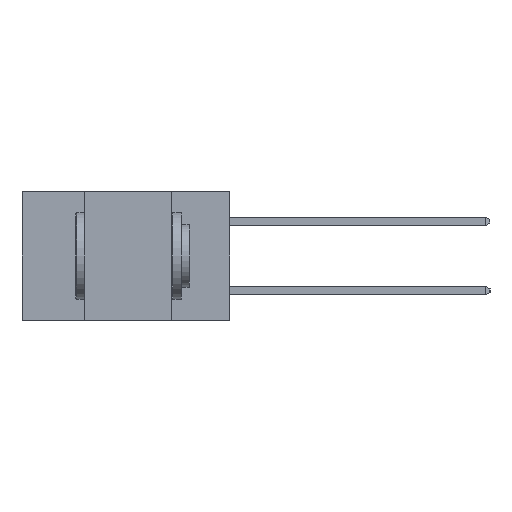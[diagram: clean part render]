
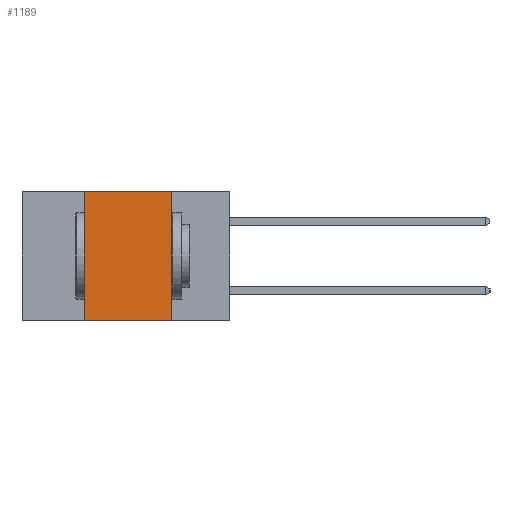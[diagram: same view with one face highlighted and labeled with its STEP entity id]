
A CAD part, left-side view. The second image highlights one B-rep face of the part: STEP entity #1189.
In plain terms, the highlighted planar face has unit normal (-1, 0, 0).
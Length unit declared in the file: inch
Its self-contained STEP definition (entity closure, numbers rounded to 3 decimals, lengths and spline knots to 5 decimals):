
#81 = PLANE ( 'NONE',  #7124 ) ;
#119 = VECTOR ( 'NONE', #3051, 39.37008 ) ;
#1189 = ADVANCED_FACE ( 'NONE', ( #8420 ), #81, .F. ) ;
#1396 = CARTESIAN_POINT ( 'NONE',  ( 0., 0.42, 0. ) ) ;
#1532 = CARTESIAN_POINT ( 'NONE',  ( 0., 0.42, -0.37 ) ) ;
#1767 = CARTESIAN_POINT ( 'NONE',  ( 0., 0.42, -0.37 ) ) ;
#2162 = LINE ( 'NONE', #2356, #16603 ) ;
#2356 = CARTESIAN_POINT ( 'NONE',  ( 0., 0.6, -0.37 ) ) ;
#3051 = DIRECTION ( 'NONE',  ( 0., 0., 1. ) ) ;
#4381 = CARTESIAN_POINT ( 'NONE',  ( 0., 0.17, -0.37 ) ) ;
#4747 = CARTESIAN_POINT ( 'NONE',  ( 0., 0.17, -0.37 ) ) ;
#5087 = LINE ( 'NONE', #9373, #15148 ) ;
#5851 = DIRECTION ( 'NONE',  ( 0., 0., -1. ) ) ;
#5996 = VERTEX_POINT ( 'NONE', #1767 ) ;
#7124 = AXIS2_PLACEMENT_3D ( 'NONE', #9971, #8505, #9987 ) ;
#7237 = VERTEX_POINT ( 'NONE', #1396 ) ;
#8259 = LINE ( 'NONE', #4381, #15367 ) ;
#8420 = FACE_OUTER_BOUND ( 'NONE', #13849, .T. ) ;
#8505 = DIRECTION ( 'NONE',  ( 1., 0., 0. ) ) ;
#8555 = EDGE_CURVE ( 'NONE', #5996, #16968, #2162, .T. ) ;
#8582 = ORIENTED_EDGE ( 'NONE', *, *, #8555, .T. ) ;
#8781 = ORIENTED_EDGE ( 'NONE', *, *, #18236, .F. ) ;
#8839 = ORIENTED_EDGE ( 'NONE', *, *, #16520, .F. ) ;
#8929 = ORIENTED_EDGE ( 'NONE', *, *, #15544, .F. ) ;
#9373 = CARTESIAN_POINT ( 'NONE',  ( 0., 0.6, 0. ) ) ;
#9971 = CARTESIAN_POINT ( 'NONE',  ( 0., 0.6, 0. ) ) ;
#9987 = DIRECTION ( 'NONE',  ( 0., 0., -1. ) ) ;
#10791 = DIRECTION ( 'NONE',  ( 0., -1., 0. ) ) ;
#13849 = EDGE_LOOP ( 'NONE', ( #8929, #8839, #8781, #8582 ) ) ;
#15148 = VECTOR ( 'NONE', #10791, 39.37008 ) ;
#15367 = VECTOR ( 'NONE', #5851, 39.37008 ) ;
#15503 = LINE ( 'NONE', #1532, #119 ) ;
#15544 = EDGE_CURVE ( 'NONE', #15692, #16968, #8259, .T. ) ;
#15692 = VERTEX_POINT ( 'NONE', #17546 ) ;
#16520 = EDGE_CURVE ( 'NONE', #7237, #15692, #5087, .T. ) ;
#16603 = VECTOR ( 'NONE', #16780, 39.37008 ) ;
#16780 = DIRECTION ( 'NONE',  ( 0., -1., 0. ) ) ;
#16968 = VERTEX_POINT ( 'NONE', #4747 ) ;
#17546 = CARTESIAN_POINT ( 'NONE',  ( 0., 0.17, 0. ) ) ;
#18236 = EDGE_CURVE ( 'NONE', #5996, #7237, #15503, .T. ) ;
